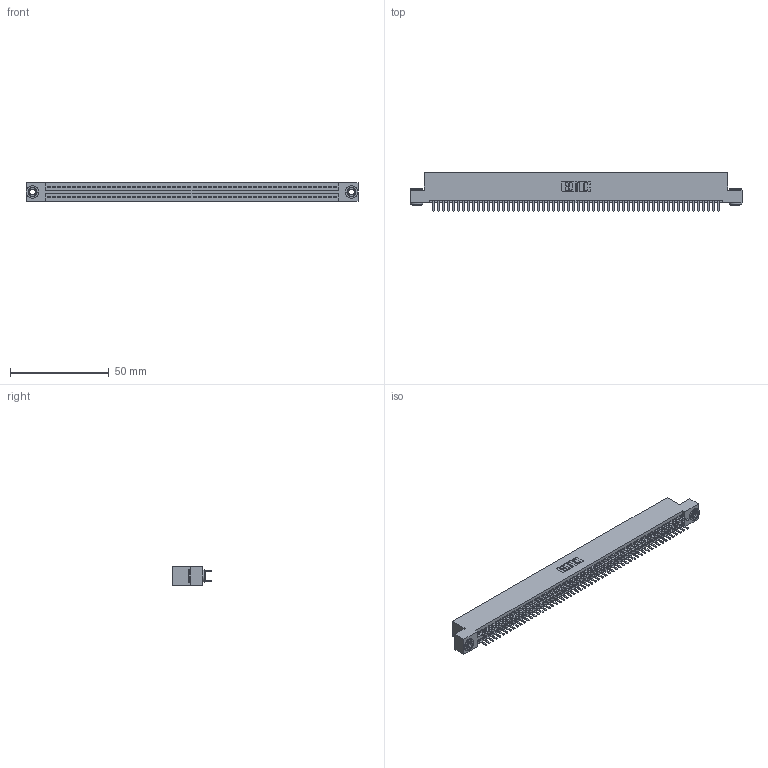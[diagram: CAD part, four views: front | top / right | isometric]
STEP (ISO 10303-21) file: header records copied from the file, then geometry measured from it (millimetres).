
FILE_DESCRIPTION (( 'STEP AP203' ), '1' );
FILE_NAME ('345-116-520-203.STEP', '2019-11-05T13:49:22', ( '' ), ( '' ), 'SwSTEP 2.0', 'SolidWorks 2016', '' );
FILE_SCHEMA (( 'CONFIG_CONTROL_DESIGN' ));
Length unit declared in the file: inch
Products named in the file (4): 345-292-001_345-293-120; 345 Part_Flush Mounting Lugs - 0.156 Dia-TH; 345-116-520-203; 345-250-002_345-250-002-102
Assembly tree (119 placements, depth 2):
  345-116-520-203
    345 Part_Flush Mounting Lugs - 0.156 Dia-TH
    345-292-001_345-293-120  x116
    345-250-002_345-250-002-102  x2
Bounding box: 168.53 x 19.68 x 9.4 mm (x, y, z)
Volume: 16488 mm3; surface area: 24778.3 mm2
Topology: 119 solids, 119 shells, 6428 faces, 18629 edges, 12106 vertices
Faces by surface type: plane 4150, cylinder 2270, cone 8
Entity records: 44118 total; most frequent: CARTESIAN_POINT 7367, ORIENTED_EDGE 7282, DIRECTION 6495, EDGE_CURVE 3641, VECTOR 3249, LINE 3249, VERTEX_POINT 2422, AXIS2_PLACEMENT_3D 1623
